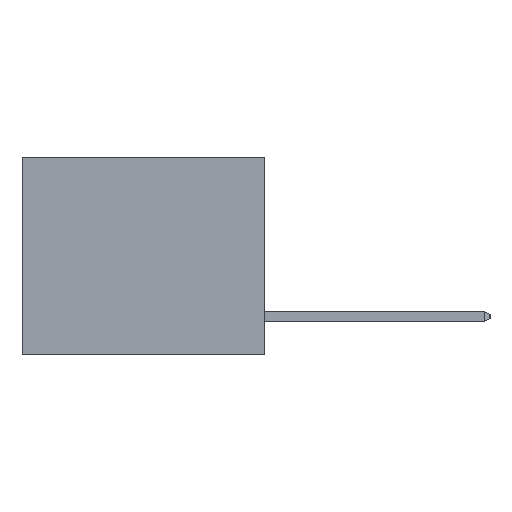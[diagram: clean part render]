
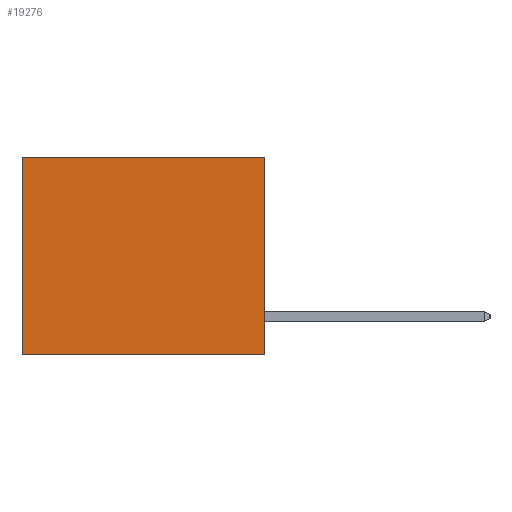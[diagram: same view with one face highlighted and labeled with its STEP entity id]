
A CAD part, left-side view. The second image highlights one B-rep face of the part: STEP entity #19276.
In plain terms, the highlighted planar face has unit normal (-1, 0, 0).
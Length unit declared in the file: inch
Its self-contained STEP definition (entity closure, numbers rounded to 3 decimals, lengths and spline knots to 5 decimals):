
#1844 = CARTESIAN_POINT ( 'NONE',  ( 0.3165, 0., -0.49 ) ) ;
#1903 = VERTEX_POINT ( 'NONE', #8412 ) ;
#2784 = PLANE ( 'NONE',  #4936 ) ;
#3904 = VERTEX_POINT ( 'NONE', #21581 ) ;
#4582 = ORIENTED_EDGE ( 'NONE', *, *, #13547, .F. ) ;
#4751 = DIRECTION ( 'NONE',  ( 0., 0., -1. ) ) ;
#4875 = VECTOR ( 'NONE', #17428, 39.37008 ) ;
#4936 = AXIS2_PLACEMENT_3D ( 'NONE', #16466, #22503, #4751 ) ;
#5025 = CARTESIAN_POINT ( 'NONE',  ( 0.3165, 0., 0. ) ) ;
#5580 = EDGE_LOOP ( 'NONE', ( #8737, #4582, #10467, #6058 ) ) ;
#5679 = DIRECTION ( 'NONE',  ( 0., 1., 0. ) ) ;
#6058 = ORIENTED_EDGE ( 'NONE', *, *, #19825, .T. ) ;
#7034 = VERTEX_POINT ( 'NONE', #5025 ) ;
#7331 = LINE ( 'NONE', #9538, #4875 ) ;
#8412 = CARTESIAN_POINT ( 'NONE',  ( 0.3165, 0.6, 0. ) ) ;
#8737 = ORIENTED_EDGE ( 'NONE', *, *, #13197, .T. ) ;
#9538 = CARTESIAN_POINT ( 'NONE',  ( 0.3165, 0., 0. ) ) ;
#9587 = VECTOR ( 'NONE', #23220, 39.37008 ) ;
#9610 = VECTOR ( 'NONE', #5679, 39.37008 ) ;
#9638 = LINE ( 'NONE', #15898, #11494 ) ;
#10467 = ORIENTED_EDGE ( 'NONE', *, *, #14165, .F. ) ;
#10591 = VERTEX_POINT ( 'NONE', #24492 ) ;
#11494 = VECTOR ( 'NONE', #20043, 39.37008 ) ;
#12905 = FACE_OUTER_BOUND ( 'NONE', #5580, .T. ) ;
#13197 = EDGE_CURVE ( 'NONE', #1903, #3904, #9638, .T. ) ;
#13270 = CARTESIAN_POINT ( 'NONE',  ( 0.3165, 0., -0.49 ) ) ;
#13547 = EDGE_CURVE ( 'NONE', #10591, #3904, #20378, .T. ) ;
#14165 = EDGE_CURVE ( 'NONE', #7034, #10591, #16945, .T. ) ;
#15898 = CARTESIAN_POINT ( 'NONE',  ( 0.3165, 0.6, -0.49 ) ) ;
#16466 = CARTESIAN_POINT ( 'NONE',  ( 0.3165, 0., -0.49 ) ) ;
#16945 = LINE ( 'NONE', #13270, #9587 ) ;
#17428 = DIRECTION ( 'NONE',  ( 0., 1., 0. ) ) ;
#19276 = ADVANCED_FACE ( 'NONE', ( #12905 ), #2784, .F. ) ;
#19825 = EDGE_CURVE ( 'NONE', #7034, #1903, #7331, .T. ) ;
#20043 = DIRECTION ( 'NONE',  ( 0., 0., -1. ) ) ;
#20378 = LINE ( 'NONE', #1844, #9610 ) ;
#21581 = CARTESIAN_POINT ( 'NONE',  ( 0.3165, 0.6, -0.49 ) ) ;
#22503 = DIRECTION ( 'NONE',  ( 1., 0., 0. ) ) ;
#23220 = DIRECTION ( 'NONE',  ( 0., 0., -1. ) ) ;
#24492 = CARTESIAN_POINT ( 'NONE',  ( 0.3165, 0., -0.49 ) ) ;
